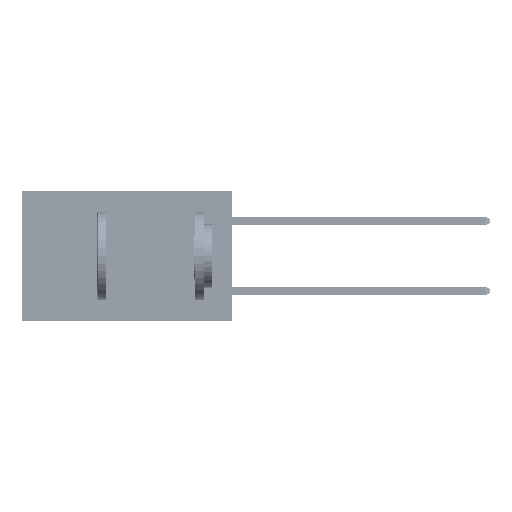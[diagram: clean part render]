
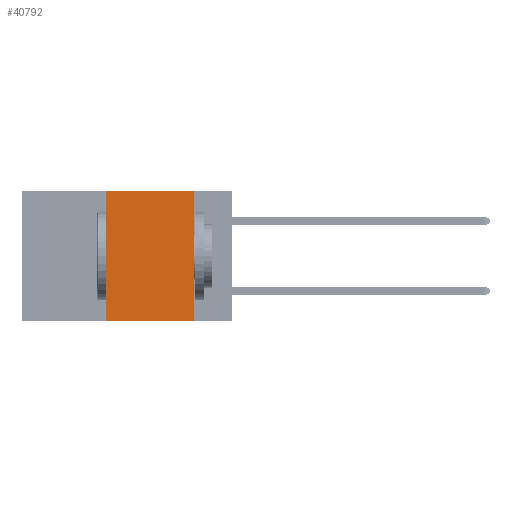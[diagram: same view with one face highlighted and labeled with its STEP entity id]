
A CAD part, left-side view. The second image highlights one B-rep face of the part: STEP entity #40792.
In plain terms, the highlighted planar face has unit normal (-1, 0, 0).
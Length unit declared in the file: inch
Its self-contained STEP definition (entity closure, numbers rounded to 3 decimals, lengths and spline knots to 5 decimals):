
#1989 = VECTOR ( 'NONE', #22569, 39.37008 ) ;
#3463 = CARTESIAN_POINT ( 'NONE',  ( 0., 0.11, -0.37 ) ) ;
#3587 = CARTESIAN_POINT ( 'NONE',  ( 0., 0.36, 0. ) ) ;
#4434 = ORIENTED_EDGE ( 'NONE', *, *, #43694, .F. ) ;
#4641 = EDGE_LOOP ( 'NONE', ( #40505, #20719, #4434, #21372 ) ) ;
#5296 = EDGE_CURVE ( 'NONE', #33620, #37510, #28150, .T. ) ;
#6920 = VECTOR ( 'NONE', #27415, 39.37008 ) ;
#7601 = DIRECTION ( 'NONE',  ( 0., 0., 1. ) ) ;
#8569 = DIRECTION ( 'NONE',  ( 0., 0., -1. ) ) ;
#8823 = VECTOR ( 'NONE', #7601, 39.37008 ) ;
#10590 = DIRECTION ( 'NONE',  ( 0., 0., -1. ) ) ;
#11665 = LINE ( 'NONE', #30439, #51203 ) ;
#12110 = VERTEX_POINT ( 'NONE', #3463 ) ;
#12311 = CARTESIAN_POINT ( 'NONE',  ( 0., 0.11, 0. ) ) ;
#13874 = LINE ( 'NONE', #50086, #1989 ) ;
#16721 = VERTEX_POINT ( 'NONE', #29761 ) ;
#19209 = EDGE_CURVE ( 'NONE', #37510, #12110, #11665, .T. ) ;
#20719 = ORIENTED_EDGE ( 'NONE', *, *, #5296, .F. ) ;
#21372 = ORIENTED_EDGE ( 'NONE', *, *, #23798, .T. ) ;
#22569 = DIRECTION ( 'NONE',  ( 0., -1., 0. ) ) ;
#23798 = EDGE_CURVE ( 'NONE', #16721, #12110, #13874, .T. ) ;
#24441 = PLANE ( 'NONE',  #32002 ) ;
#27415 = DIRECTION ( 'NONE',  ( 0., -1., 0. ) ) ;
#28150 = LINE ( 'NONE', #50974, #6920 ) ;
#28411 = CARTESIAN_POINT ( 'NONE',  ( 0., 0.6, 0. ) ) ;
#29761 = CARTESIAN_POINT ( 'NONE',  ( 0., 0.36, -0.37 ) ) ;
#30020 = LINE ( 'NONE', #3587, #8823 ) ;
#30439 = CARTESIAN_POINT ( 'NONE',  ( 0., 0.11, 0. ) ) ;
#32002 = AXIS2_PLACEMENT_3D ( 'NONE', #28411, #32374, #8569 ) ;
#32374 = DIRECTION ( 'NONE',  ( 1., 0., 0. ) ) ;
#33620 = VERTEX_POINT ( 'NONE', #34972 ) ;
#34972 = CARTESIAN_POINT ( 'NONE',  ( 0., 0.36, 0. ) ) ;
#37510 = VERTEX_POINT ( 'NONE', #12311 ) ;
#40505 = ORIENTED_EDGE ( 'NONE', *, *, #19209, .F. ) ;
#40792 = ADVANCED_FACE ( 'NONE', ( #40803 ), #24441, .F. ) ;
#40803 = FACE_OUTER_BOUND ( 'NONE', #4641, .T. ) ;
#43694 = EDGE_CURVE ( 'NONE', #16721, #33620, #30020, .T. ) ;
#50086 = CARTESIAN_POINT ( 'NONE',  ( 0., 0.6, -0.37 ) ) ;
#50974 = CARTESIAN_POINT ( 'NONE',  ( 0., 0.6, 0. ) ) ;
#51203 = VECTOR ( 'NONE', #10590, 39.37008 ) ;
